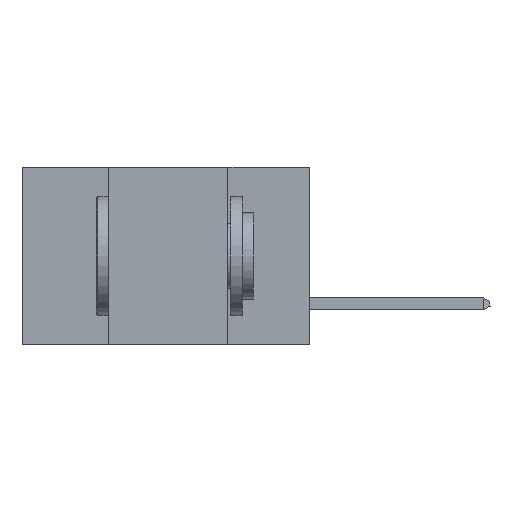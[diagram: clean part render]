
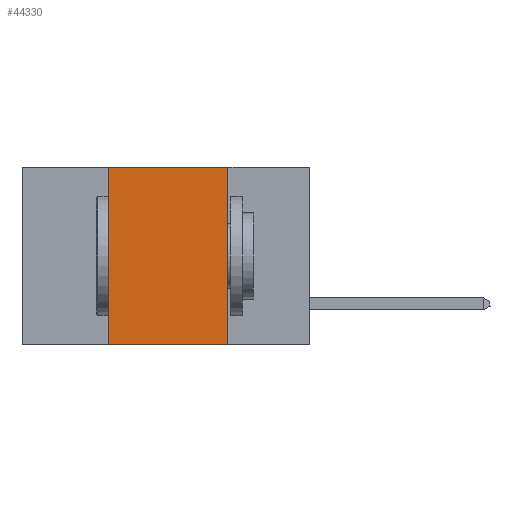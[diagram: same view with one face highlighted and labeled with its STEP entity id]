
A CAD part, left-side view. The second image highlights one B-rep face of the part: STEP entity #44330.
In plain terms, the highlighted planar face has unit normal (-1, 0, 0).
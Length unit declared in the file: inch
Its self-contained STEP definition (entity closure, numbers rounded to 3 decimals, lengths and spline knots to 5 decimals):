
#2235 = VECTOR ( 'NONE', #45108, 39.37008 ) ;
#2410 = VERTEX_POINT ( 'NONE', #41028 ) ;
#3557 = LINE ( 'NONE', #25038, #31151 ) ;
#4340 = PLANE ( 'NONE',  #34226 ) ;
#5622 = CARTESIAN_POINT ( 'NONE',  ( 0., 0.6, -0.37 ) ) ;
#6529 = EDGE_CURVE ( 'NONE', #2410, #40755, #3557, .T. ) ;
#6768 = LINE ( 'NONE', #5622, #2235 ) ;
#10067 = EDGE_CURVE ( 'NONE', #19303, #38188, #6768, .T. ) ;
#10769 = CARTESIAN_POINT ( 'NONE',  ( 0., 0.17, 0. ) ) ;
#12983 = EDGE_CURVE ( 'NONE', #19303, #2410, #41359, .T. ) ;
#15582 = LINE ( 'NONE', #10769, #29110 ) ;
#16132 = DIRECTION ( 'NONE',  ( 0., -1., 0. ) ) ;
#18354 = CARTESIAN_POINT ( 'NONE',  ( 0., 0.42, -0.37 ) ) ;
#18643 = CARTESIAN_POINT ( 'NONE',  ( 0., 0.6, 0. ) ) ;
#19303 = VERTEX_POINT ( 'NONE', #18354 ) ;
#19437 = ORIENTED_EDGE ( 'NONE', *, *, #12983, .F. ) ;
#25038 = CARTESIAN_POINT ( 'NONE',  ( 0., 0.6, 0. ) ) ;
#25835 = ORIENTED_EDGE ( 'NONE', *, *, #6529, .F. ) ;
#26550 = CARTESIAN_POINT ( 'NONE',  ( 0., 0.42, 0. ) ) ;
#29110 = VECTOR ( 'NONE', #31904, 39.37008 ) ;
#30667 = VECTOR ( 'NONE', #33794, 39.37008 ) ;
#31151 = VECTOR ( 'NONE', #16132, 39.37008 ) ;
#31332 = CARTESIAN_POINT ( 'NONE',  ( 0., 0.17, -0.37 ) ) ;
#31904 = DIRECTION ( 'NONE',  ( 0., 0., -1. ) ) ;
#32933 = ORIENTED_EDGE ( 'NONE', *, *, #45812, .F. ) ;
#32965 = CARTESIAN_POINT ( 'NONE',  ( 0., 0.17, 0. ) ) ;
#33794 = DIRECTION ( 'NONE',  ( 0., 0., 1. ) ) ;
#34226 = AXIS2_PLACEMENT_3D ( 'NONE', #18643, #43995, #43668 ) ;
#35407 = ORIENTED_EDGE ( 'NONE', *, *, #10067, .T. ) ;
#38188 = VERTEX_POINT ( 'NONE', #31332 ) ;
#40755 = VERTEX_POINT ( 'NONE', #32965 ) ;
#41028 = CARTESIAN_POINT ( 'NONE',  ( 0., 0.42, 0. ) ) ;
#41359 = LINE ( 'NONE', #26550, #30667 ) ;
#42344 = EDGE_LOOP ( 'NONE', ( #32933, #25835, #19437, #35407 ) ) ;
#43668 = DIRECTION ( 'NONE',  ( 0., 0., -1. ) ) ;
#43995 = DIRECTION ( 'NONE',  ( 1., 0., 0. ) ) ;
#44330 = ADVANCED_FACE ( 'NONE', ( #45571 ), #4340, .F. ) ;
#45108 = DIRECTION ( 'NONE',  ( 0., -1., 0. ) ) ;
#45571 = FACE_OUTER_BOUND ( 'NONE', #42344, .T. ) ;
#45812 = EDGE_CURVE ( 'NONE', #40755, #38188, #15582, .T. ) ;
